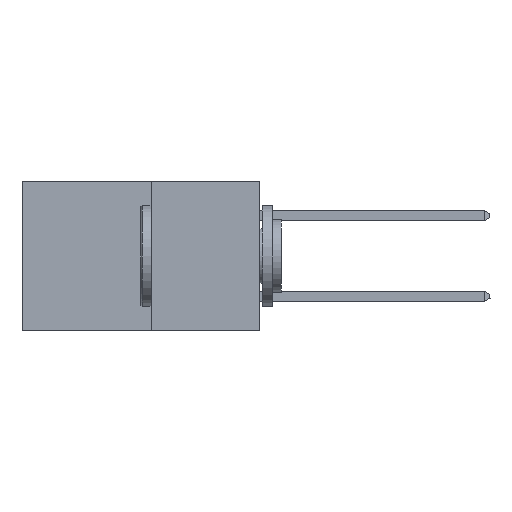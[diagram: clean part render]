
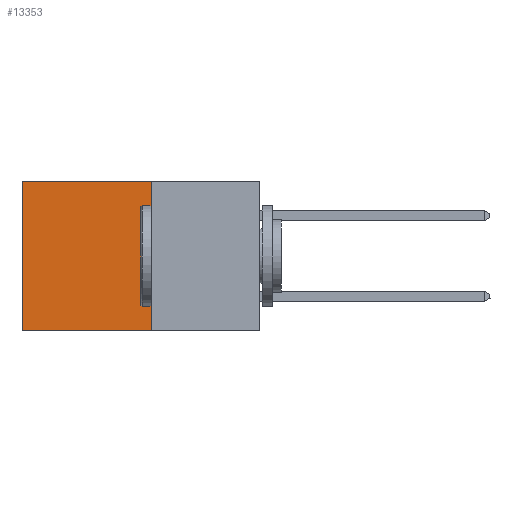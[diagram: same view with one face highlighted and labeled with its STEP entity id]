
A CAD part, left-side view. The second image highlights one B-rep face of the part: STEP entity #13353.
In plain terms, the highlighted planar face has unit normal (-1, 0, 0).
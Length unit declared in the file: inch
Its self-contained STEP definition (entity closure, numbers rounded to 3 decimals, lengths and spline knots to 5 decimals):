
#99 = ORIENTED_EDGE ( 'NONE', *, *, #18295, .F. ) ;
#455 = DIRECTION ( 'NONE',  ( 0., 1., 0. ) ) ;
#651 = DIRECTION ( 'NONE',  ( 1., 0., 0. ) ) ;
#1321 = ORIENTED_EDGE ( 'NONE', *, *, #8474, .T. ) ;
#2044 = CARTESIAN_POINT ( 'NONE',  ( 0.277, 0.59, 0. ) ) ;
#2981 = CARTESIAN_POINT ( 'NONE',  ( 0.277, 0.59, -0.37 ) ) ;
#3691 = CARTESIAN_POINT ( 'NONE',  ( 0.277, 0.27, -0.37 ) ) ;
#5526 = DIRECTION ( 'NONE',  ( 0., 0., -1. ) ) ;
#5813 = EDGE_LOOP ( 'NONE', ( #12285, #99, #10691, #1321 ) ) ;
#6029 = PLANE ( 'NONE',  #20563 ) ;
#7420 = VERTEX_POINT ( 'NONE', #2981 ) ;
#7870 = CARTESIAN_POINT ( 'NONE',  ( 0.277, 0.27, -0.37 ) ) ;
#8339 = EDGE_CURVE ( 'NONE', #12720, #16527, #16094, .T. ) ;
#8474 = EDGE_CURVE ( 'NONE', #12720, #20225, #13812, .T. ) ;
#8955 = VECTOR ( 'NONE', #21067, 39.37008 ) ;
#9831 = FACE_OUTER_BOUND ( 'NONE', #5813, .T. ) ;
#10691 = ORIENTED_EDGE ( 'NONE', *, *, #8339, .F. ) ;
#11277 = VECTOR ( 'NONE', #5526, 39.37008 ) ;
#12078 = LINE ( 'NONE', #14795, #16906 ) ;
#12285 = ORIENTED_EDGE ( 'NONE', *, *, #18647, .T. ) ;
#12446 = CARTESIAN_POINT ( 'NONE',  ( 0.277, 0.27, -0.37 ) ) ;
#12720 = VERTEX_POINT ( 'NONE', #22631 ) ;
#13111 = CARTESIAN_POINT ( 'NONE',  ( 0.277, 0.27, 0. ) ) ;
#13303 = DIRECTION ( 'NONE',  ( 0., 0., -1. ) ) ;
#13353 = ADVANCED_FACE ( 'NONE', ( #9831 ), #6029, .F. ) ;
#13812 = LINE ( 'NONE', #13111, #18072 ) ;
#14795 = CARTESIAN_POINT ( 'NONE',  ( 0.277, 0.27, -0.37 ) ) ;
#16094 = LINE ( 'NONE', #3691, #11277 ) ;
#16527 = VERTEX_POINT ( 'NONE', #12446 ) ;
#16639 = DIRECTION ( 'NONE',  ( 0., 1., 0. ) ) ;
#16906 = VECTOR ( 'NONE', #16639, 39.37008 ) ;
#18072 = VECTOR ( 'NONE', #455, 39.37008 ) ;
#18295 = EDGE_CURVE ( 'NONE', #16527, #7420, #12078, .T. ) ;
#18647 = EDGE_CURVE ( 'NONE', #20225, #7420, #23447, .T. ) ;
#19246 = CARTESIAN_POINT ( 'NONE',  ( 0.277, 0.59, -0.37 ) ) ;
#20225 = VERTEX_POINT ( 'NONE', #2044 ) ;
#20563 = AXIS2_PLACEMENT_3D ( 'NONE', #7870, #651, #13303 ) ;
#21067 = DIRECTION ( 'NONE',  ( 0., 0., -1. ) ) ;
#22631 = CARTESIAN_POINT ( 'NONE',  ( 0.277, 0.27, 0. ) ) ;
#23447 = LINE ( 'NONE', #19246, #8955 ) ;
